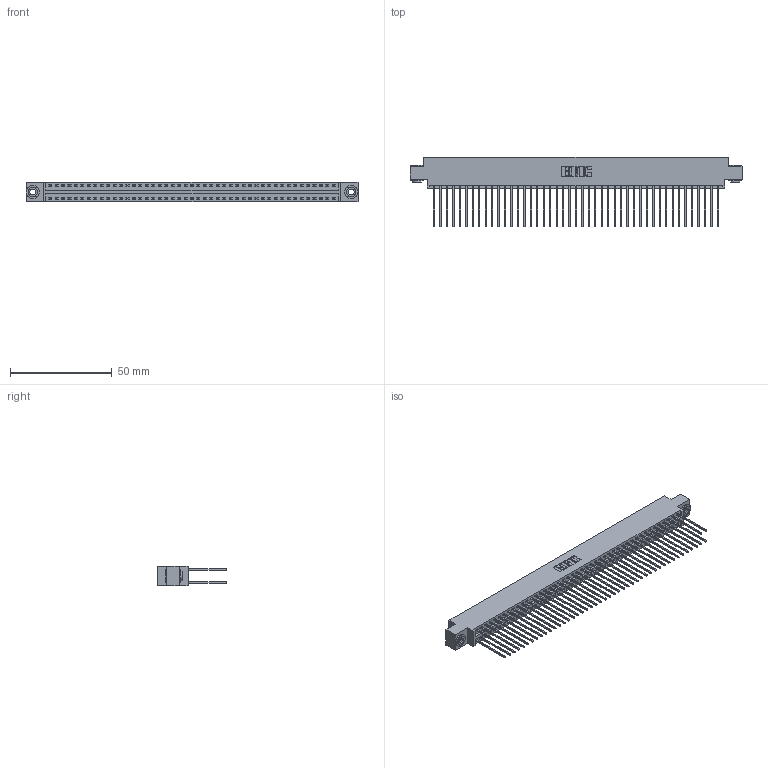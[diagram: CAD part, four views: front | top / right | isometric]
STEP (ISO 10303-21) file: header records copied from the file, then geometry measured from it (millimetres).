
FILE_DESCRIPTION (( 'STEP AP203' ), '1' );
FILE_NAME ('396-090-541-803.STEP', '2019-11-02T15:34:08', ( '' ), ( '' ), 'SwSTEP 2.0', 'SolidWorks 2016', '' );
FILE_SCHEMA (( 'CONFIG_CONTROL_DESIGN' ));
Length unit declared in the file: inch
Products named in the file (4): 346 Part_0.170 Offset - 0.156 Dia-TH; 345-292-001_345-293-141; 345-250-002_345-250-002-102; 396-090-541-803
Assembly tree (93 placements, depth 2):
  396-090-541-803
    346 Part_0.170 Offset - 0.156 Dia-TH
    345-292-001_345-293-141  x90
    345-250-002_345-250-002-102  x2
Bounding box: 163.45 x 34.29 x 9.4 mm (x, y, z)
Volume: 16342.7 mm3; surface area: 25381.4 mm2
Topology: 93 solids, 93 shells, 4844 faces, 14367 edges, 9454 vertices
Faces by surface type: plane 3240, cylinder 1596, cone 8
Entity records: 29764 total; most frequent: CARTESIAN_POINT 4879, ORIENTED_EDGE 4806, DIRECTION 4381, EDGE_CURVE 2403, LINE 2067, VECTOR 2067, VERTEX_POINT 1598, AXIS2_PLACEMENT_3D 1157
